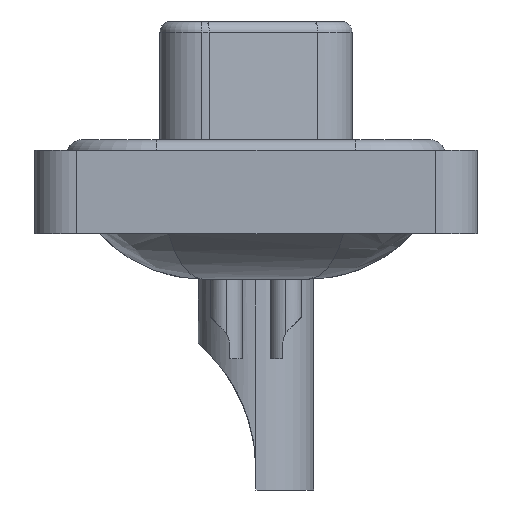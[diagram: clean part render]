
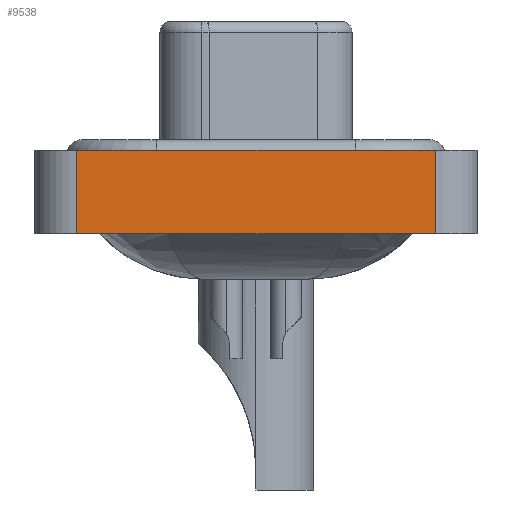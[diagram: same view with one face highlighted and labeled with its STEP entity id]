
A CAD part, left-side view. The second image highlights one B-rep face of the part: STEP entity #9538.
In plain terms, the highlighted planar face has unit normal (-1, 0, 0).
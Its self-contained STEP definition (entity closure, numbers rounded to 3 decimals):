
#599 = VERTEX_POINT ( 'NONE', #14288 ) ;
#912 = EDGE_LOOP ( 'NONE', ( #24244, #12118, #10323, #8324 ) ) ;
#1218 = VECTOR ( 'NONE', #4504, 1000. ) ;
#2869 = CARTESIAN_POINT ( 'NONE',  ( -7.35, -8.55, 0.4 ) ) ;
#3537 = LINE ( 'NONE', #18965, #19559 ) ;
#4504 = DIRECTION ( 'NONE',  ( 0., -1., 0. ) ) ;
#5786 = AXIS2_PLACEMENT_3D ( 'NONE', #21402, #11561, #6001 ) ;
#5903 = CARTESIAN_POINT ( 'NONE',  ( -7.35, 8.55, -3.6 ) ) ;
#6001 = DIRECTION ( 'NONE',  ( 0., 0., 1. ) ) ;
#6223 = CARTESIAN_POINT ( 'NONE',  ( -7.35, -8.55, -3.6 ) ) ;
#6283 = EDGE_CURVE ( 'NONE', #9500, #16437, #19322, .T. ) ;
#7781 = CARTESIAN_POINT ( 'NONE',  ( -7.35, -8.55, -3.6 ) ) ;
#8324 = ORIENTED_EDGE ( 'NONE', *, *, #15044, .T. ) ;
#8501 = EDGE_CURVE ( 'NONE', #599, #16437, #9638, .T. ) ;
#9500 = VERTEX_POINT ( 'NONE', #21039 ) ;
#9538 = ADVANCED_FACE ( 'NONE', ( #22895 ), #11808, .T. ) ;
#9638 = LINE ( 'NONE', #7781, #12073 ) ;
#10323 = ORIENTED_EDGE ( 'NONE', *, *, #14406, .F. ) ;
#11561 = DIRECTION ( 'NONE',  ( -1., 0., 0. ) ) ;
#11808 = PLANE ( 'NONE',  #5786 ) ;
#12073 = VECTOR ( 'NONE', #13226, 1000. ) ;
#12118 = ORIENTED_EDGE ( 'NONE', *, *, #6283, .F. ) ;
#13226 = DIRECTION ( 'NONE',  ( 0., 0., 1. ) ) ;
#14288 = CARTESIAN_POINT ( 'NONE',  ( -7.35, -8.55, -3.6 ) ) ;
#14406 = EDGE_CURVE ( 'NONE', #20228, #9500, #3537, .T. ) ;
#14909 = DIRECTION ( 'NONE',  ( 0., 0., 1. ) ) ;
#15044 = EDGE_CURVE ( 'NONE', #20228, #599, #23107, .T. ) ;
#15361 = DIRECTION ( 'NONE',  ( 0., -1., 0. ) ) ;
#16437 = VERTEX_POINT ( 'NONE', #2869 ) ;
#17111 = VECTOR ( 'NONE', #15361, 1000. ) ;
#17711 = CARTESIAN_POINT ( 'NONE',  ( -7.35, -8.55, 0.4 ) ) ;
#18965 = CARTESIAN_POINT ( 'NONE',  ( -7.35, 8.55, -3.6 ) ) ;
#19322 = LINE ( 'NONE', #17711, #1218 ) ;
#19559 = VECTOR ( 'NONE', #14909, 1000. ) ;
#20228 = VERTEX_POINT ( 'NONE', #5903 ) ;
#21039 = CARTESIAN_POINT ( 'NONE',  ( -7.35, 8.55, 0.4 ) ) ;
#21402 = CARTESIAN_POINT ( 'NONE',  ( -7.35, -8.55, -3.6 ) ) ;
#22895 = FACE_OUTER_BOUND ( 'NONE', #912, .T. ) ;
#23107 = LINE ( 'NONE', #6223, #17111 ) ;
#24244 = ORIENTED_EDGE ( 'NONE', *, *, #8501, .T. ) ;
